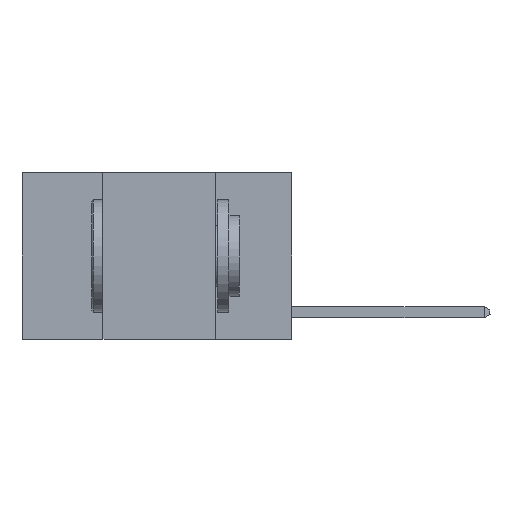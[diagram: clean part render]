
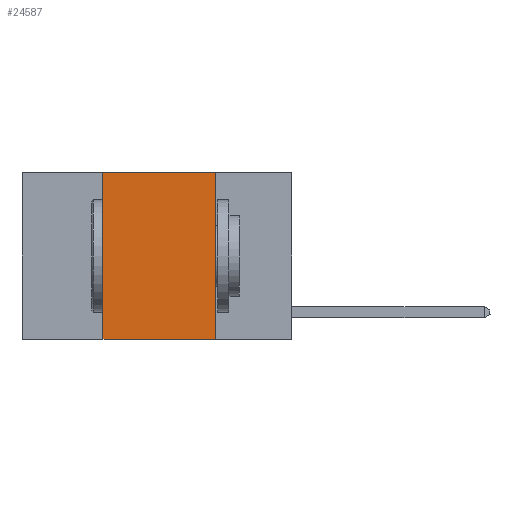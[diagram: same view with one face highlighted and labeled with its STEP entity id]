
A CAD part, left-side view. The second image highlights one B-rep face of the part: STEP entity #24587.
In plain terms, the highlighted planar face has unit normal (-1, 0, 0).
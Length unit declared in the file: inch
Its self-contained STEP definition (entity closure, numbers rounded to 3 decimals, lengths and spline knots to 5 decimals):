
#583 = AXIS2_PLACEMENT_3D ( 'NONE', #2487, #10196, #10328 ) ;
#899 = DIRECTION ( 'NONE',  ( 0., 0., 1. ) ) ;
#1294 = VERTEX_POINT ( 'NONE', #16543 ) ;
#2135 = ORIENTED_EDGE ( 'NONE', *, *, #16010, .F. ) ;
#2487 = CARTESIAN_POINT ( 'NONE',  ( 0., 0.6, 0. ) ) ;
#2886 = DIRECTION ( 'NONE',  ( 0., -1., 0. ) ) ;
#3153 = LINE ( 'NONE', #20975, #16151 ) ;
#3864 = EDGE_LOOP ( 'NONE', ( #19549, #2135, #10419, #3993 ) ) ;
#3990 = CARTESIAN_POINT ( 'NONE',  ( 0., 0.6, 0. ) ) ;
#3993 = ORIENTED_EDGE ( 'NONE', *, *, #7913, .T. ) ;
#4862 = CARTESIAN_POINT ( 'NONE',  ( 0., 0.17, 0. ) ) ;
#5600 = DIRECTION ( 'NONE',  ( 0., 0., -1. ) ) ;
#6194 = VERTEX_POINT ( 'NONE', #4862 ) ;
#6989 = CARTESIAN_POINT ( 'NONE',  ( 0., 0.17, -0.37 ) ) ;
#7913 = EDGE_CURVE ( 'NONE', #10101, #10702, #3153, .T. ) ;
#10101 = VERTEX_POINT ( 'NONE', #19621 ) ;
#10196 = DIRECTION ( 'NONE',  ( 1., 0., 0. ) ) ;
#10328 = DIRECTION ( 'NONE',  ( 0., 0., -1. ) ) ;
#10419 = ORIENTED_EDGE ( 'NONE', *, *, #20354, .F. ) ;
#10702 = VERTEX_POINT ( 'NONE', #6989 ) ;
#11115 = VECTOR ( 'NONE', #899, 39.37008 ) ;
#13911 = PLANE ( 'NONE',  #583 ) ;
#15202 = LINE ( 'NONE', #17240, #15723 ) ;
#15723 = VECTOR ( 'NONE', #5600, 39.37008 ) ;
#16010 = EDGE_CURVE ( 'NONE', #1294, #6194, #25012, .T. ) ;
#16151 = VECTOR ( 'NONE', #2886, 39.37008 ) ;
#16543 = CARTESIAN_POINT ( 'NONE',  ( 0., 0.42, 0. ) ) ;
#17240 = CARTESIAN_POINT ( 'NONE',  ( 0., 0.17, 0. ) ) ;
#17741 = FACE_OUTER_BOUND ( 'NONE', #3864, .T. ) ;
#18206 = LINE ( 'NONE', #24389, #11115 ) ;
#19549 = ORIENTED_EDGE ( 'NONE', *, *, #24498, .F. ) ;
#19621 = CARTESIAN_POINT ( 'NONE',  ( 0., 0.42, -0.37 ) ) ;
#20354 = EDGE_CURVE ( 'NONE', #10101, #1294, #18206, .T. ) ;
#20460 = VECTOR ( 'NONE', #21168, 39.37008 ) ;
#20975 = CARTESIAN_POINT ( 'NONE',  ( 0., 0.6, -0.37 ) ) ;
#21168 = DIRECTION ( 'NONE',  ( 0., -1., 0. ) ) ;
#24389 = CARTESIAN_POINT ( 'NONE',  ( 0., 0.42, 0. ) ) ;
#24498 = EDGE_CURVE ( 'NONE', #6194, #10702, #15202, .T. ) ;
#24587 = ADVANCED_FACE ( 'NONE', ( #17741 ), #13911, .F. ) ;
#25012 = LINE ( 'NONE', #3990, #20460 ) ;
